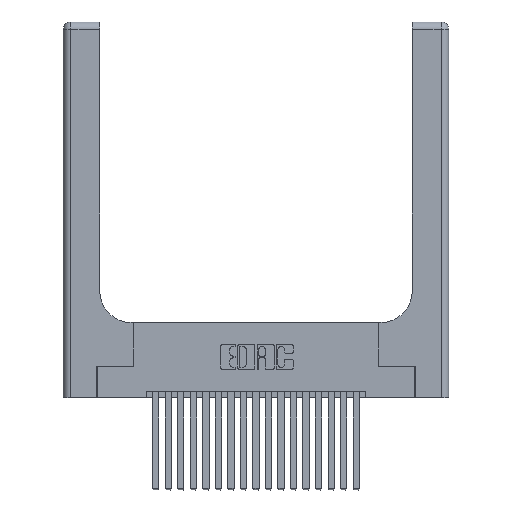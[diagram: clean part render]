
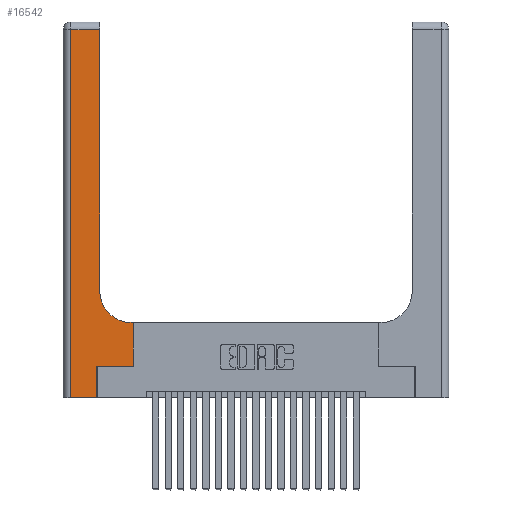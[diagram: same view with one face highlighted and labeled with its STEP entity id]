
A CAD part, top view. The second image highlights one B-rep face of the part: STEP entity #16542.
In plain terms, the highlighted planar face has unit normal (0, 0, 1).
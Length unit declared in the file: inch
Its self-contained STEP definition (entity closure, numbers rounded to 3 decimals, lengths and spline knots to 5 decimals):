
#64 = VERTEX_POINT ( 'NONE', #11348 ) ;
#701 = ORIENTED_EDGE ( 'NONE', *, *, #2917, .T. ) ;
#830 = VERTEX_POINT ( 'NONE', #15975 ) ;
#1074 = DIRECTION ( 'NONE',  ( -1., 0., 0. ) ) ;
#1128 = CARTESIAN_POINT ( 'NONE',  ( 0.2915, 0.85, 0.37 ) ) ;
#1266 = LINE ( 'NONE', #2773, #10330 ) ;
#1763 = DIRECTION ( 'NONE',  ( 1., 0., 0. ) ) ;
#2411 = EDGE_CURVE ( 'NONE', #12996, #17297, #8927, .T. ) ;
#2457 = VERTEX_POINT ( 'NONE', #13535 ) ;
#2773 = CARTESIAN_POINT ( 'NONE',  ( 0.269, 0.25, 0.37 ) ) ;
#2907 = DIRECTION ( 'NONE',  ( 1., 0., 0. ) ) ;
#2917 = EDGE_CURVE ( 'NONE', #64, #20587, #1266, .T. ) ;
#3082 = DIRECTION ( 'NONE',  ( 0., 1., 0. ) ) ;
#3522 = CARTESIAN_POINT ( 'NONE',  ( 0.06, 3., 0.37 ) ) ;
#3637 = VECTOR ( 'NONE', #15362, 39.37008 ) ;
#3791 = LINE ( 'NONE', #3522, #21065 ) ;
#4071 = LINE ( 'NONE', #4443, #20828 ) ;
#4086 = VECTOR ( 'NONE', #1074, 39.37008 ) ;
#4443 = CARTESIAN_POINT ( 'NONE',  ( 0.2915, 3., 0.37 ) ) ;
#4470 = DIRECTION ( 'NONE',  ( 0., 0., -1. ) ) ;
#5154 = ORIENTED_EDGE ( 'NONE', *, *, #16562, .T. ) ;
#5329 = LINE ( 'NONE', #13629, #18677 ) ;
#6190 = CARTESIAN_POINT ( 'NONE',  ( 0.2915, 0.6, 0.37 ) ) ;
#6324 = VECTOR ( 'NONE', #20068, 39.37008 ) ;
#7337 = ORIENTED_EDGE ( 'NONE', *, *, #19039, .T. ) ;
#7816 = CARTESIAN_POINT ( 'NONE',  ( 0., 3., 0.37 ) ) ;
#8604 = LINE ( 'NONE', #6190, #4086 ) ;
#8927 = CIRCLE ( 'NONE', #20770, 0.25 ) ;
#9080 = CARTESIAN_POINT ( 'NONE',  ( 0.5415, 0.6, 0.37 ) ) ;
#9136 = FACE_OUTER_BOUND ( 'NONE', #13772, .T. ) ;
#9538 = DIRECTION ( 'NONE',  ( 0., 1., 0. ) ) ;
#9696 = CARTESIAN_POINT ( 'NONE',  ( 0.5585, 0.6, 0.37 ) ) ;
#9824 = ORIENTED_EDGE ( 'NONE', *, *, #21072, .T. ) ;
#9998 = CARTESIAN_POINT ( 'NONE',  ( 0.5415, 0.85, 0.37 ) ) ;
#10220 = VERTEX_POINT ( 'NONE', #15007 ) ;
#10240 = ORIENTED_EDGE ( 'NONE', *, *, #11081, .T. ) ;
#10275 = DIRECTION ( 'NONE',  ( 0., -1., 0. ) ) ;
#10330 = VECTOR ( 'NONE', #2907, 39.37008 ) ;
#10493 = CARTESIAN_POINT ( 'NONE',  ( 0.5585, 0.25, 0.37 ) ) ;
#10527 = ORIENTED_EDGE ( 'NONE', *, *, #21199, .T. ) ;
#11081 = EDGE_CURVE ( 'NONE', #17297, #2457, #4071, .T. ) ;
#11342 = EDGE_CURVE ( 'NONE', #15542, #830, #3791, .T. ) ;
#11348 = CARTESIAN_POINT ( 'NONE',  ( 0.269, 0.25, 0.37 ) ) ;
#12633 = LINE ( 'NONE', #20353, #3637 ) ;
#12996 = VERTEX_POINT ( 'NONE', #9080 ) ;
#13535 = CARTESIAN_POINT ( 'NONE',  ( 0.2915, 2.94, 0.37 ) ) ;
#13629 = CARTESIAN_POINT ( 'NONE',  ( 0., 0., 0.37 ) ) ;
#13772 = EDGE_LOOP ( 'NONE', ( #10240, #10527, #19073, #7337, #9824, #701, #17177, #5154, #14013 ) ) ;
#14013 = ORIENTED_EDGE ( 'NONE', *, *, #2411, .T. ) ;
#14520 = DIRECTION ( 'NONE',  ( 1., 0., 0. ) ) ;
#14539 = DIRECTION ( 'NONE',  ( 0., 0., -1. ) ) ;
#15007 = CARTESIAN_POINT ( 'NONE',  ( 0.269, 0., 0.37 ) ) ;
#15253 = LINE ( 'NONE', #16754, #6324 ) ;
#15267 = AXIS2_PLACEMENT_3D ( 'NONE', #7816, #4470, #16254 ) ;
#15362 = DIRECTION ( 'NONE',  ( -1., 0., 0. ) ) ;
#15542 = VERTEX_POINT ( 'NONE', #18735 ) ;
#15975 = CARTESIAN_POINT ( 'NONE',  ( 0.06, 0., 0.37 ) ) ;
#16254 = DIRECTION ( 'NONE',  ( -1., 0., 0. ) ) ;
#16542 = ADVANCED_FACE ( 'NONE', ( #9136 ), #19487, .F. ) ;
#16562 = EDGE_CURVE ( 'NONE', #21520, #12996, #8604, .T. ) ;
#16754 = CARTESIAN_POINT ( 'NONE',  ( 0.269, 0., 0.37 ) ) ;
#17175 = VECTOR ( 'NONE', #3082, 39.37008 ) ;
#17177 = ORIENTED_EDGE ( 'NONE', *, *, #18182, .T. ) ;
#17297 = VERTEX_POINT ( 'NONE', #1128 ) ;
#18170 = CARTESIAN_POINT ( 'NONE',  ( 0.5585, 0.25, 0.37 ) ) ;
#18182 = EDGE_CURVE ( 'NONE', #20587, #21520, #21531, .T. ) ;
#18677 = VECTOR ( 'NONE', #1763, 39.37008 ) ;
#18735 = CARTESIAN_POINT ( 'NONE',  ( 0.06, 2.94, 0.37 ) ) ;
#19039 = EDGE_CURVE ( 'NONE', #830, #10220, #5329, .T. ) ;
#19073 = ORIENTED_EDGE ( 'NONE', *, *, #11342, .T. ) ;
#19487 = PLANE ( 'NONE',  #15267 ) ;
#20068 = DIRECTION ( 'NONE',  ( 0., 1., 0. ) ) ;
#20353 = CARTESIAN_POINT ( 'NONE',  ( 0., 2.94, 0.37 ) ) ;
#20587 = VERTEX_POINT ( 'NONE', #10493 ) ;
#20770 = AXIS2_PLACEMENT_3D ( 'NONE', #9998, #14539, #14520 ) ;
#20828 = VECTOR ( 'NONE', #9538, 39.37008 ) ;
#21065 = VECTOR ( 'NONE', #10275, 39.37008 ) ;
#21072 = EDGE_CURVE ( 'NONE', #10220, #64, #15253, .T. ) ;
#21199 = EDGE_CURVE ( 'NONE', #2457, #15542, #12633, .T. ) ;
#21520 = VERTEX_POINT ( 'NONE', #9696 ) ;
#21531 = LINE ( 'NONE', #18170, #17175 ) ;
